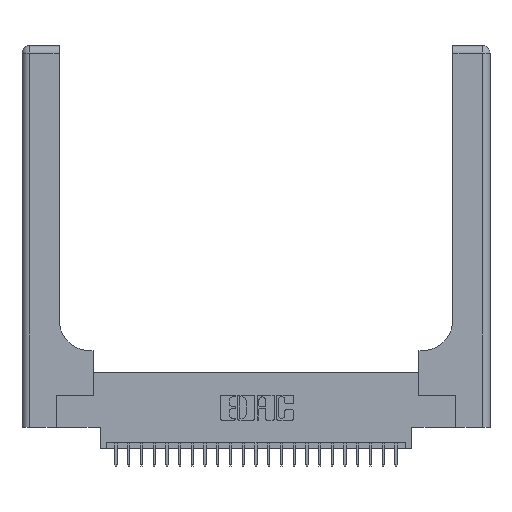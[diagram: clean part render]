
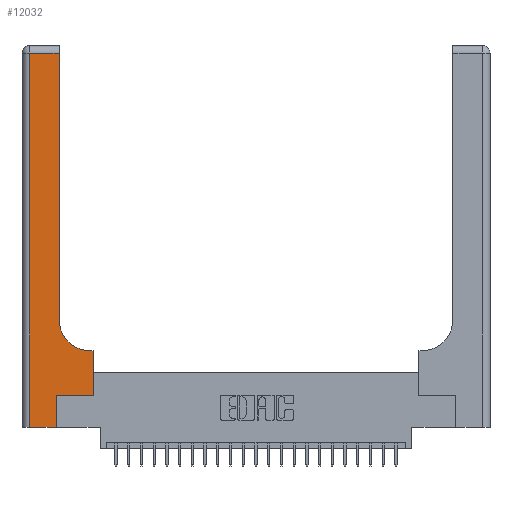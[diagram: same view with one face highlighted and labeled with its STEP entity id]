
A CAD part, top view. The second image highlights one B-rep face of the part: STEP entity #12032.
In plain terms, the highlighted planar face has unit normal (0, 0, 1).
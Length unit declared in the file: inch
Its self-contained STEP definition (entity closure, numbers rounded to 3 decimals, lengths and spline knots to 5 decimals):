
#464 = ORIENTED_EDGE ( 'NONE', *, *, #18191, .T. ) ;
#637 = CARTESIAN_POINT ( 'NONE',  ( 0., 0., 0.37 ) ) ;
#929 = AXIS2_PLACEMENT_3D ( 'NONE', #21696, #21318, #19242 ) ;
#1942 = VERTEX_POINT ( 'NONE', #19447 ) ;
#1949 = VECTOR ( 'NONE', #12267, 39.37008 ) ;
#2723 = PLANE ( 'NONE',  #6591 ) ;
#3202 = DIRECTION ( 'NONE',  ( 1., 0., 0. ) ) ;
#3364 = EDGE_CURVE ( 'NONE', #24010, #22958, #7823, .T. ) ;
#3595 = VECTOR ( 'NONE', #23910, 39.37008 ) ;
#3651 = CARTESIAN_POINT ( 'NONE',  ( 0.269, 0.25, 0.37 ) ) ;
#4166 = ORIENTED_EDGE ( 'NONE', *, *, #12682, .T. ) ;
#4204 = VERTEX_POINT ( 'NONE', #5218 ) ;
#4276 = CARTESIAN_POINT ( 'NONE',  ( 0.2915, 0.6, 0.37 ) ) ;
#4425 = CARTESIAN_POINT ( 'NONE',  ( 0., 2.94, 0.37 ) ) ;
#5218 = CARTESIAN_POINT ( 'NONE',  ( 0.5415, 0.6, 0.37 ) ) ;
#5546 = CARTESIAN_POINT ( 'NONE',  ( 0.5585, 0.25, 0.37 ) ) ;
#5685 = LINE ( 'NONE', #17562, #13488 ) ;
#5710 = LINE ( 'NONE', #13731, #8290 ) ;
#6101 = CARTESIAN_POINT ( 'NONE',  ( 0.5585, 0.6, 0.37 ) ) ;
#6142 = DIRECTION ( 'NONE',  ( 0., 0., -1. ) ) ;
#6174 = DIRECTION ( 'NONE',  ( 0., 1., 0. ) ) ;
#6543 = CARTESIAN_POINT ( 'NONE',  ( 0.2915, 0.85, 0.37 ) ) ;
#6591 = AXIS2_PLACEMENT_3D ( 'NONE', #18802, #6142, #20247 ) ;
#7781 = VERTEX_POINT ( 'NONE', #17571 ) ;
#7823 = LINE ( 'NONE', #11539, #3595 ) ;
#8092 = VERTEX_POINT ( 'NONE', #17937 ) ;
#8290 = VECTOR ( 'NONE', #25942, 39.37008 ) ;
#9553 = VECTOR ( 'NONE', #11995, 39.37008 ) ;
#11539 = CARTESIAN_POINT ( 'NONE',  ( 0.2915, 3., 0.37 ) ) ;
#11612 = VECTOR ( 'NONE', #6174, 39.37008 ) ;
#11995 = DIRECTION ( 'NONE',  ( 1., 0., 0. ) ) ;
#12032 = ADVANCED_FACE ( 'NONE', ( #12690 ), #2723, .F. ) ;
#12120 = ORIENTED_EDGE ( 'NONE', *, *, #3364, .T. ) ;
#12267 = DIRECTION ( 'NONE',  ( -1., 0., 0. ) ) ;
#12338 = EDGE_CURVE ( 'NONE', #14216, #4204, #22288, .T. ) ;
#12340 = ORIENTED_EDGE ( 'NONE', *, *, #23299, .T. ) ;
#12682 = EDGE_CURVE ( 'NONE', #1942, #14216, #22083, .T. ) ;
#12690 = FACE_OUTER_BOUND ( 'NONE', #12781, .T. ) ;
#12705 = ORIENTED_EDGE ( 'NONE', *, *, #22250, .T. ) ;
#12781 = EDGE_LOOP ( 'NONE', ( #12120, #12705, #14067, #464, #17598, #15786, #4166, #20797, #12340 ) ) ;
#13488 = VECTOR ( 'NONE', #3202, 39.37008 ) ;
#13731 = CARTESIAN_POINT ( 'NONE',  ( 0.269, 0., 0.37 ) ) ;
#13935 = VECTOR ( 'NONE', #22575, 39.37008 ) ;
#14067 = ORIENTED_EDGE ( 'NONE', *, *, #16166, .T. ) ;
#14216 = VERTEX_POINT ( 'NONE', #6101 ) ;
#15450 = CARTESIAN_POINT ( 'NONE',  ( 0.2915, 2.94, 0.37 ) ) ;
#15786 = ORIENTED_EDGE ( 'NONE', *, *, #21694, .T. ) ;
#16166 = EDGE_CURVE ( 'NONE', #7781, #8092, #22297, .T. ) ;
#16559 = LINE ( 'NONE', #4425, #13935 ) ;
#17282 = VERTEX_POINT ( 'NONE', #21218 ) ;
#17562 = CARTESIAN_POINT ( 'NONE',  ( 0.269, 0.25, 0.37 ) ) ;
#17571 = CARTESIAN_POINT ( 'NONE',  ( 0.06, 2.94, 0.37 ) ) ;
#17598 = ORIENTED_EDGE ( 'NONE', *, *, #18230, .T. ) ;
#17792 = CIRCLE ( 'NONE', #929, 0.25 ) ;
#17937 = CARTESIAN_POINT ( 'NONE',  ( 0.06, 0., 0.37 ) ) ;
#18191 = EDGE_CURVE ( 'NONE', #8092, #17282, #22140, .T. ) ;
#18230 = EDGE_CURVE ( 'NONE', #17282, #23945, #5710, .T. ) ;
#18672 = DIRECTION ( 'NONE',  ( 0., -1., 0. ) ) ;
#18802 = CARTESIAN_POINT ( 'NONE',  ( 0., 3., 0.37 ) ) ;
#19242 = DIRECTION ( 'NONE',  ( 1., 0., 0. ) ) ;
#19447 = CARTESIAN_POINT ( 'NONE',  ( 0.5585, 0.25, 0.37 ) ) ;
#20247 = DIRECTION ( 'NONE',  ( -1., 0., 0. ) ) ;
#20553 = VECTOR ( 'NONE', #18672, 39.37008 ) ;
#20635 = CARTESIAN_POINT ( 'NONE',  ( 0.06, 3., 0.37 ) ) ;
#20797 = ORIENTED_EDGE ( 'NONE', *, *, #12338, .T. ) ;
#21218 = CARTESIAN_POINT ( 'NONE',  ( 0.269, 0., 0.37 ) ) ;
#21318 = DIRECTION ( 'NONE',  ( 0., 0., -1. ) ) ;
#21694 = EDGE_CURVE ( 'NONE', #23945, #1942, #5685, .T. ) ;
#21696 = CARTESIAN_POINT ( 'NONE',  ( 0.5415, 0.85, 0.37 ) ) ;
#22083 = LINE ( 'NONE', #5546, #11612 ) ;
#22140 = LINE ( 'NONE', #637, #9553 ) ;
#22250 = EDGE_CURVE ( 'NONE', #22958, #7781, #16559, .T. ) ;
#22288 = LINE ( 'NONE', #4276, #1949 ) ;
#22297 = LINE ( 'NONE', #20635, #20553 ) ;
#22575 = DIRECTION ( 'NONE',  ( -1., 0., 0. ) ) ;
#22958 = VERTEX_POINT ( 'NONE', #15450 ) ;
#23299 = EDGE_CURVE ( 'NONE', #4204, #24010, #17792, .T. ) ;
#23910 = DIRECTION ( 'NONE',  ( 0., 1., 0. ) ) ;
#23945 = VERTEX_POINT ( 'NONE', #3651 ) ;
#24010 = VERTEX_POINT ( 'NONE', #6543 ) ;
#25942 = DIRECTION ( 'NONE',  ( 0., 1., 0. ) ) ;
